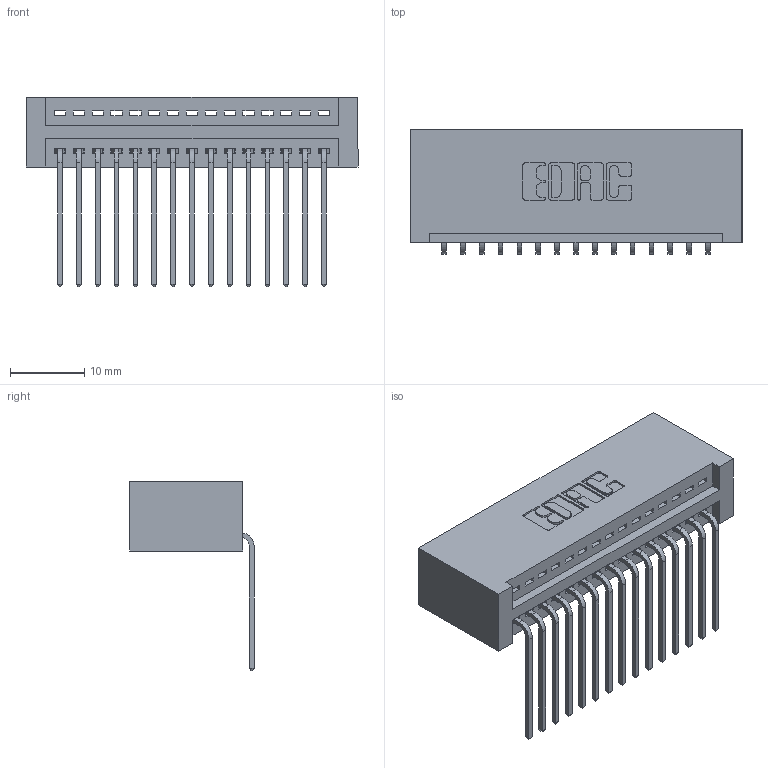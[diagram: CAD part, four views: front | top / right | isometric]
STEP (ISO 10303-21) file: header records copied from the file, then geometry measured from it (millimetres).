
FILE_DESCRIPTION (( 'STEP AP203' ), '1' );
FILE_NAME ('345-015-559-101.STEP', '2018-08-18T20:52:50', ( '' ), ( '' ), 'SwSTEP 2.0', 'SolidWorks 2016', '' );
FILE_SCHEMA (( 'CONFIG_CONTROL_DESIGN' ));
Length unit declared in the file: inch
Products named in the file (3): 345-015-559-101; 345 Part_No Mounting Lugs; 345-292-001_558 559 Tail - 1
Assembly tree (16 placements, depth 2):
  345-015-559-101
    345 Part_No Mounting Lugs
    345-292-001_558 559 Tail - 1  x15
Bounding box: 44.7 x 16.75 x 25.53 mm (x, y, z)
Volume: 4659.2 mm3; surface area: 6308.5 mm2
Topology: 16 solids, 16 shells, 1018 faces, 3047 edges, 2010 vertices
Faces by surface type: plane 706, cylinder 312
Entity records: 14731 total; most frequent: CARTESIAN_POINT 2561, ORIENTED_EDGE 2510, DIRECTION 2269, EDGE_CURVE 1255, VECTOR 1071, LINE 1071, VERTEX_POINT 834, AXIS2_PLACEMENT_3D 599
